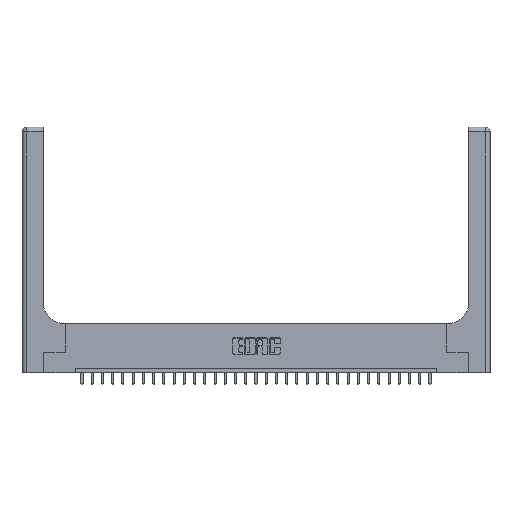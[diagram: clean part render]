
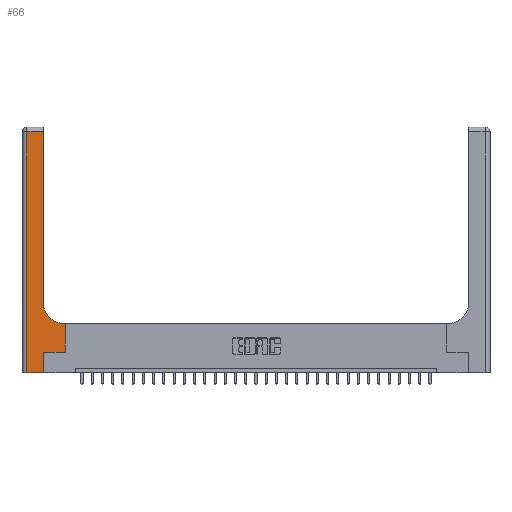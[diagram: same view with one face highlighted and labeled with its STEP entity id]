
A CAD part, top view. The second image highlights one B-rep face of the part: STEP entity #66.
In plain terms, the highlighted planar face has unit normal (0, 0, 1).
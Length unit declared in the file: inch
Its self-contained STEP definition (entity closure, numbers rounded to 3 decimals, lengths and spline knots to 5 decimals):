
#63 = EDGE_CURVE ( 'NONE', #9194, #5363, #13807, .T. ) ;
#66 = ADVANCED_FACE ( 'NONE', ( #17948 ), #19687, .F. ) ;
#124 = EDGE_CURVE ( 'NONE', #14123, #20831, #7117, .T. ) ;
#893 = EDGE_CURVE ( 'NONE', #6840, #14123, #7321, .T. ) ;
#1170 = VERTEX_POINT ( 'NONE', #8164 ) ;
#1537 = VECTOR ( 'NONE', #20110, 39.37008 ) ;
#1565 = CARTESIAN_POINT ( 'NONE',  ( 0.528, 0.25, 0.37 ) ) ;
#3830 = DIRECTION ( 'NONE',  ( 1., 0., 0. ) ) ;
#4020 = VECTOR ( 'NONE', #6612, 39.37008 ) ;
#4442 = VECTOR ( 'NONE', #27027, 39.37008 ) ;
#4749 = VECTOR ( 'NONE', #22556, 39.37008 ) ;
#4921 = AXIS2_PLACEMENT_3D ( 'NONE', #10322, #19038, #21200 ) ;
#4966 = CARTESIAN_POINT ( 'NONE',  ( 0., 3., 0.37 ) ) ;
#5321 = CARTESIAN_POINT ( 'NONE',  ( 0.26, 3., 0.37 ) ) ;
#5363 = VERTEX_POINT ( 'NONE', #21618 ) ;
#5369 = ORIENTED_EDGE ( 'NONE', *, *, #893, .T. ) ;
#6164 = ORIENTED_EDGE ( 'NONE', *, *, #6452, .T. ) ;
#6452 = EDGE_CURVE ( 'NONE', #21178, #12356, #25496, .T. ) ;
#6612 = DIRECTION ( 'NONE',  ( 0., 1., 0. ) ) ;
#6840 = VERTEX_POINT ( 'NONE', #14988 ) ;
#6961 = DIRECTION ( 'NONE',  ( -1., 0., 0. ) ) ;
#7117 = LINE ( 'NONE', #19968, #1537 ) ;
#7321 = LINE ( 'NONE', #5321, #23717 ) ;
#7403 = EDGE_LOOP ( 'NONE', ( #5369, #12652, #21471, #20307, #26004, #6164, #9190, #14456, #7783 ) ) ;
#7746 = DIRECTION ( 'NONE',  ( 0., 1., 0. ) ) ;
#7783 = ORIENTED_EDGE ( 'NONE', *, *, #10927, .T. ) ;
#8164 = CARTESIAN_POINT ( 'NONE',  ( 0.265, 0., 0.37 ) ) ;
#9190 = ORIENTED_EDGE ( 'NONE', *, *, #15902, .T. ) ;
#9194 = VERTEX_POINT ( 'NONE', #16622 ) ;
#9500 = CARTESIAN_POINT ( 'NONE',  ( 0.06, 0., 0.37 ) ) ;
#10322 = CARTESIAN_POINT ( 'NONE',  ( 0.51, 0.85, 0.37 ) ) ;
#10395 = EDGE_CURVE ( 'NONE', #1170, #21178, #23145, .T. ) ;
#10927 = EDGE_CURVE ( 'NONE', #5363, #6840, #16314, .T. ) ;
#12049 = LINE ( 'NONE', #14324, #19775 ) ;
#12356 = VERTEX_POINT ( 'NONE', #1565 ) ;
#12652 = ORIENTED_EDGE ( 'NONE', *, *, #124, .T. ) ;
#13807 = LINE ( 'NONE', #15812, #4749 ) ;
#13919 = DIRECTION ( 'NONE',  ( 0., -1., 0. ) ) ;
#14123 = VERTEX_POINT ( 'NONE', #20406 ) ;
#14252 = CARTESIAN_POINT ( 'NONE',  ( 0.265, 0.25, 0.37 ) ) ;
#14324 = CARTESIAN_POINT ( 'NONE',  ( 0.06, 3., 0.37 ) ) ;
#14431 = CARTESIAN_POINT ( 'NONE',  ( 0.06, 2.94, 0.37 ) ) ;
#14456 = ORIENTED_EDGE ( 'NONE', *, *, #63, .T. ) ;
#14988 = CARTESIAN_POINT ( 'NONE',  ( 0.26, 0.85, 0.37 ) ) ;
#15386 = DIRECTION ( 'NONE',  ( 0., 0., -1. ) ) ;
#15812 = CARTESIAN_POINT ( 'NONE',  ( 0.26, 0.6, 0.37 ) ) ;
#15902 = EDGE_CURVE ( 'NONE', #12356, #9194, #17438, .T. ) ;
#16314 = CIRCLE ( 'NONE', #4921, 0.25 ) ;
#16622 = CARTESIAN_POINT ( 'NONE',  ( 0.528, 0.6, 0.37 ) ) ;
#16892 = EDGE_CURVE ( 'NONE', #20831, #24038, #12049, .T. ) ;
#17438 = LINE ( 'NONE', #26208, #4020 ) ;
#17948 = FACE_OUTER_BOUND ( 'NONE', #7403, .T. ) ;
#18835 = LINE ( 'NONE', #25313, #19327 ) ;
#19038 = DIRECTION ( 'NONE',  ( 0., 0., -1. ) ) ;
#19051 = EDGE_CURVE ( 'NONE', #24038, #1170, #18835, .T. ) ;
#19327 = VECTOR ( 'NONE', #3830, 39.37008 ) ;
#19687 = PLANE ( 'NONE',  #26216 ) ;
#19775 = VECTOR ( 'NONE', #13919, 39.37008 ) ;
#19968 = CARTESIAN_POINT ( 'NONE',  ( 0., 2.94, 0.37 ) ) ;
#20110 = DIRECTION ( 'NONE',  ( -1., 0., 0. ) ) ;
#20307 = ORIENTED_EDGE ( 'NONE', *, *, #19051, .T. ) ;
#20406 = CARTESIAN_POINT ( 'NONE',  ( 0.26, 2.94, 0.37 ) ) ;
#20831 = VERTEX_POINT ( 'NONE', #14431 ) ;
#21119 = CARTESIAN_POINT ( 'NONE',  ( 0.265, 0., 0.37 ) ) ;
#21178 = VERTEX_POINT ( 'NONE', #14252 ) ;
#21191 = DIRECTION ( 'NONE',  ( 1., 0., 0. ) ) ;
#21200 = DIRECTION ( 'NONE',  ( 1., 0., 0. ) ) ;
#21471 = ORIENTED_EDGE ( 'NONE', *, *, #16892, .T. ) ;
#21618 = CARTESIAN_POINT ( 'NONE',  ( 0.51, 0.6, 0.37 ) ) ;
#22442 = VECTOR ( 'NONE', #21191, 39.37008 ) ;
#22556 = DIRECTION ( 'NONE',  ( -1., 0., 0. ) ) ;
#23145 = LINE ( 'NONE', #21119, #4442 ) ;
#23717 = VECTOR ( 'NONE', #7746, 39.37008 ) ;
#24038 = VERTEX_POINT ( 'NONE', #9500 ) ;
#25313 = CARTESIAN_POINT ( 'NONE',  ( 0., 0., 0.37 ) ) ;
#25496 = LINE ( 'NONE', #28229, #22442 ) ;
#26004 = ORIENTED_EDGE ( 'NONE', *, *, #10395, .T. ) ;
#26208 = CARTESIAN_POINT ( 'NONE',  ( 0.528, 0.25, 0.37 ) ) ;
#26216 = AXIS2_PLACEMENT_3D ( 'NONE', #4966, #15386, #6961 ) ;
#27027 = DIRECTION ( 'NONE',  ( 0., 1., 0. ) ) ;
#28229 = CARTESIAN_POINT ( 'NONE',  ( 0.265, 0.25, 0.37 ) ) ;
